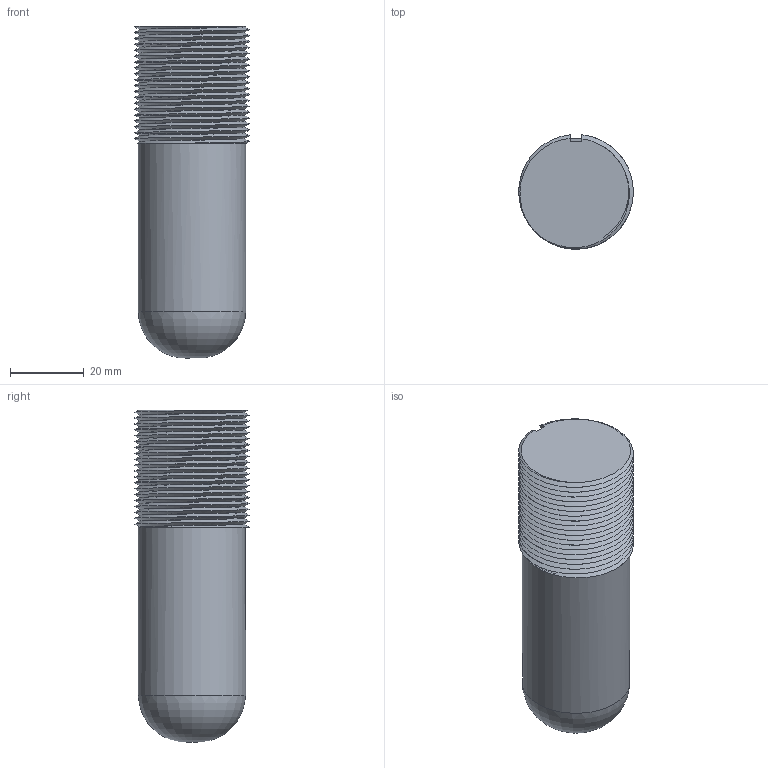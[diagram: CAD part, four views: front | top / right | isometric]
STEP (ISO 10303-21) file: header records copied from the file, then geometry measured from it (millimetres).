
FILE_DESCRIPTION (( 'STEP AP214' ), '1' );
FILE_NAME ('False_Buffer_Stubby.STEP', '2014-02-12T13:36:36', ( 'elpi' ), ( '' ), 'SwSTEP 2.0', 'SolidWorks 2013', '' );
FILE_SCHEMA (( 'AUTOMOTIVE_DESIGN' ));
Length unit declared in the file: inch
Products named in the file (1): False_Buffer_Stubby
Bounding box: 31.01 x 30.92 x 89.9 mm (x, y, z)
Volume: 57889.1 mm3; surface area: 11700.5 mm2
Topology: 1 solids, 1 shells, 90 faces, 335 edges, 247 vertices
Faces by surface type: bspline 60, cylinder 22, plane 7, torus 1
Full cylindrical faces by diameter (mm): 29.083 x1
Entity records: 49680 total; most frequent: CARTESIAN_POINT 47708, ORIENTED_EDGE 664, EDGE_CURVE 332, VERTEX_POINT 246, DIRECTION 124, B_SPLINE_CURVE_WITH_KNOTS 117, EDGE_LOOP 92, FACE_OUTER_BOUND 92
